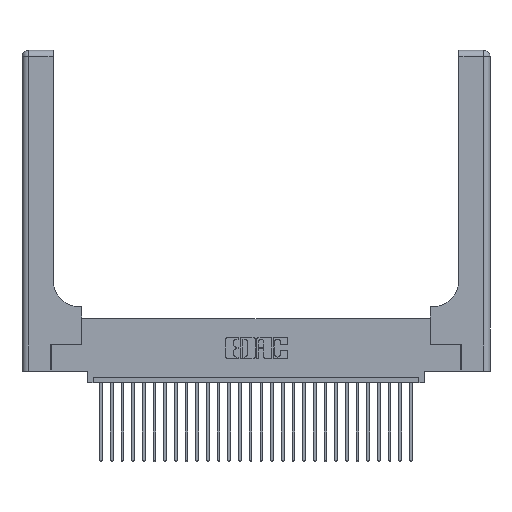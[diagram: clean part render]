
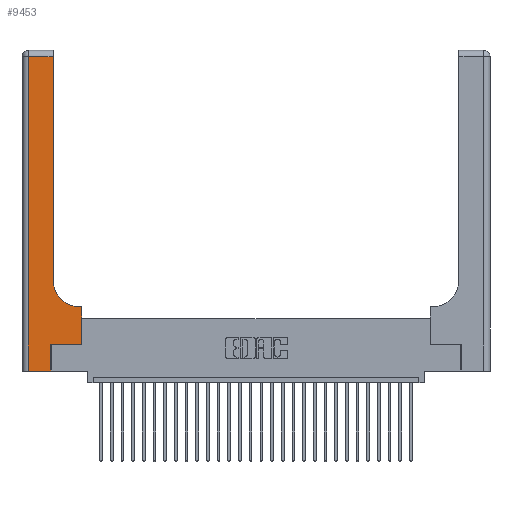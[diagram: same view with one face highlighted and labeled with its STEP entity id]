
A CAD part, top view. The second image highlights one B-rep face of the part: STEP entity #9453.
In plain terms, the highlighted planar face has unit normal (0, 0, 1).
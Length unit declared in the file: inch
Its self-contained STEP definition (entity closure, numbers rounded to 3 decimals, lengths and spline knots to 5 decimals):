
#142 = AXIS2_PLACEMENT_3D ( 'NONE', #19046, #7745, #23716 ) ;
#339 = CARTESIAN_POINT ( 'NONE',  ( 0.269, 0.25, 0.37 ) ) ;
#976 = CARTESIAN_POINT ( 'NONE',  ( 0.06, 0., 0.37 ) ) ;
#1400 = ORIENTED_EDGE ( 'NONE', *, *, #13694, .T. ) ;
#2178 = DIRECTION ( 'NONE',  ( 0., 1., 0. ) ) ;
#2209 = CARTESIAN_POINT ( 'NONE',  ( 0.2915, 0.85, 0.37 ) ) ;
#4068 = DIRECTION ( 'NONE',  ( 0., -1., 0. ) ) ;
#4505 = LINE ( 'NONE', #11571, #14521 ) ;
#4667 = VERTEX_POINT ( 'NONE', #976 ) ;
#4817 = EDGE_LOOP ( 'NONE', ( #17429, #28504, #21119, #14970, #29357, #1400, #16852, #25524, #18754 ) ) ;
#5330 = VERTEX_POINT ( 'NONE', #7600 ) ;
#5729 = PLANE ( 'NONE',  #28825 ) ;
#5917 = CARTESIAN_POINT ( 'NONE',  ( 0.06, 2.94, 0.37 ) ) ;
#6837 = LINE ( 'NONE', #26134, #29347 ) ;
#7389 = EDGE_CURVE ( 'NONE', #4667, #15415, #9346, .T. ) ;
#7600 = CARTESIAN_POINT ( 'NONE',  ( 0.269, 0.25, 0.37 ) ) ;
#7728 = CARTESIAN_POINT ( 'NONE',  ( 0.2915, 0.6, 0.37 ) ) ;
#7737 = VERTEX_POINT ( 'NONE', #13306 ) ;
#7745 = DIRECTION ( 'NONE',  ( 0., 0., -1. ) ) ;
#8053 = CARTESIAN_POINT ( 'NONE',  ( 0., 3., 0.37 ) ) ;
#8600 = VERTEX_POINT ( 'NONE', #13179 ) ;
#8840 = EDGE_CURVE ( 'NONE', #15415, #5330, #6837, .T. ) ;
#8973 = CIRCLE ( 'NONE', #142, 0.25 ) ;
#9220 = LINE ( 'NONE', #28189, #25616 ) ;
#9346 = LINE ( 'NONE', #27579, #26835 ) ;
#9453 = ADVANCED_FACE ( 'NONE', ( #23609 ), #5729, .F. ) ;
#9780 = EDGE_CURVE ( 'NONE', #8600, #21674, #12906, .T. ) ;
#10156 = EDGE_CURVE ( 'NONE', #15222, #7737, #22520, .T. ) ;
#10460 = DIRECTION ( 'NONE',  ( 0., 0., -1. ) ) ;
#10884 = LINE ( 'NONE', #24831, #17646 ) ;
#11571 = CARTESIAN_POINT ( 'NONE',  ( 0.5585, 0.25, 0.37 ) ) ;
#11700 = VERTEX_POINT ( 'NONE', #2209 ) ;
#11926 = EDGE_CURVE ( 'NONE', #11700, #8600, #9220, .T. ) ;
#12906 = LINE ( 'NONE', #24669, #14345 ) ;
#13091 = VERTEX_POINT ( 'NONE', #21787 ) ;
#13179 = CARTESIAN_POINT ( 'NONE',  ( 0.2915, 2.94, 0.37 ) ) ;
#13306 = CARTESIAN_POINT ( 'NONE',  ( 0.5415, 0.6, 0.37 ) ) ;
#13457 = DIRECTION ( 'NONE',  ( -1., 0., 0. ) ) ;
#13694 = EDGE_CURVE ( 'NONE', #5330, #13091, #19827, .T. ) ;
#14055 = CARTESIAN_POINT ( 'NONE',  ( 0.5585, 0.6, 0.37 ) ) ;
#14345 = VECTOR ( 'NONE', #18057, 39.37008 ) ;
#14521 = VECTOR ( 'NONE', #2178, 39.37008 ) ;
#14680 = DIRECTION ( 'NONE',  ( 0., 1., 0. ) ) ;
#14970 = ORIENTED_EDGE ( 'NONE', *, *, #7389, .T. ) ;
#14992 = EDGE_CURVE ( 'NONE', #13091, #15222, #4505, .T. ) ;
#15222 = VERTEX_POINT ( 'NONE', #14055 ) ;
#15415 = VERTEX_POINT ( 'NONE', #26212 ) ;
#15906 = DIRECTION ( 'NONE',  ( -1., 0., 0. ) ) ;
#16852 = ORIENTED_EDGE ( 'NONE', *, *, #14992, .T. ) ;
#17277 = EDGE_CURVE ( 'NONE', #21674, #4667, #10884, .T. ) ;
#17429 = ORIENTED_EDGE ( 'NONE', *, *, #11926, .T. ) ;
#17646 = VECTOR ( 'NONE', #4068, 39.37008 ) ;
#18057 = DIRECTION ( 'NONE',  ( -1., 0., 0. ) ) ;
#18636 = DIRECTION ( 'NONE',  ( 1., 0., 0. ) ) ;
#18754 = ORIENTED_EDGE ( 'NONE', *, *, #18944, .T. ) ;
#18944 = EDGE_CURVE ( 'NONE', #7737, #11700, #8973, .T. ) ;
#19046 = CARTESIAN_POINT ( 'NONE',  ( 0.5415, 0.85, 0.37 ) ) ;
#19097 = VECTOR ( 'NONE', #18636, 39.37008 ) ;
#19827 = LINE ( 'NONE', #339, #19097 ) ;
#21003 = DIRECTION ( 'NONE',  ( 1., 0., 0. ) ) ;
#21119 = ORIENTED_EDGE ( 'NONE', *, *, #17277, .T. ) ;
#21674 = VERTEX_POINT ( 'NONE', #5917 ) ;
#21787 = CARTESIAN_POINT ( 'NONE',  ( 0.5585, 0.25, 0.37 ) ) ;
#22520 = LINE ( 'NONE', #7728, #25727 ) ;
#23609 = FACE_OUTER_BOUND ( 'NONE', #4817, .T. ) ;
#23716 = DIRECTION ( 'NONE',  ( 1., 0., 0. ) ) ;
#24669 = CARTESIAN_POINT ( 'NONE',  ( 0., 2.94, 0.37 ) ) ;
#24831 = CARTESIAN_POINT ( 'NONE',  ( 0.06, 3., 0.37 ) ) ;
#25524 = ORIENTED_EDGE ( 'NONE', *, *, #10156, .T. ) ;
#25616 = VECTOR ( 'NONE', #14680, 39.37008 ) ;
#25727 = VECTOR ( 'NONE', #15906, 39.37008 ) ;
#26134 = CARTESIAN_POINT ( 'NONE',  ( 0.269, 0., 0.37 ) ) ;
#26212 = CARTESIAN_POINT ( 'NONE',  ( 0.269, 0., 0.37 ) ) ;
#26835 = VECTOR ( 'NONE', #21003, 39.37008 ) ;
#27579 = CARTESIAN_POINT ( 'NONE',  ( 0., 0., 0.37 ) ) ;
#28189 = CARTESIAN_POINT ( 'NONE',  ( 0.2915, 3., 0.37 ) ) ;
#28488 = DIRECTION ( 'NONE',  ( 0., 1., 0. ) ) ;
#28504 = ORIENTED_EDGE ( 'NONE', *, *, #9780, .T. ) ;
#28825 = AXIS2_PLACEMENT_3D ( 'NONE', #8053, #10460, #13457 ) ;
#29347 = VECTOR ( 'NONE', #28488, 39.37008 ) ;
#29357 = ORIENTED_EDGE ( 'NONE', *, *, #8840, .T. ) ;
